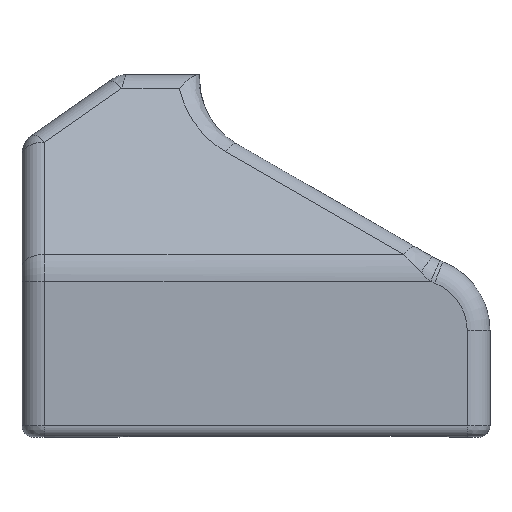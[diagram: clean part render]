
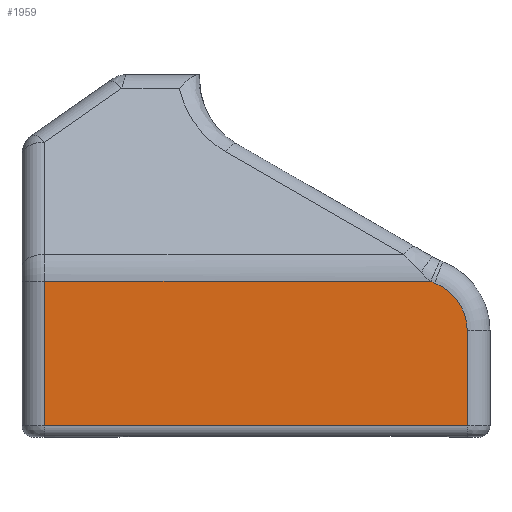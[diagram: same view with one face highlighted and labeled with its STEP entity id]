
A CAD part, left-side view. The second image highlights one B-rep face of the part: STEP entity #1959.
In plain terms, the highlighted planar face has unit normal (-1, 0, 0).
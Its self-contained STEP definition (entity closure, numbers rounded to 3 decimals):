
#72=PLANE('',#2136);
#104=LINE('',#2942,#241);
#123=LINE('',#3056,#260);
#142=LINE('',#3189,#279);
#143=LINE('',#3194,#280);
#241=VECTOR('',#2320,10.);
#260=VECTOR('',#2385,10.);
#279=VECTOR('',#2480,10.);
#280=VECTOR('',#2485,10.);
#490=FACE_OUTER_BOUND('',#613,.T.);
#613=EDGE_LOOP('',(#1442,#1443,#1444,#1445,#1446,#1447));
#750=CIRCLE('',#2137,4.5);
#751=CIRCLE('',#2138,8.5);
#826=VERTEX_POINT('',#2926);
#830=VERTEX_POINT('',#2940);
#857=VERTEX_POINT('',#3055);
#883=VERTEX_POINT('',#3188);
#884=VERTEX_POINT('',#3190);
#885=VERTEX_POINT('',#3192);
#1013=EDGE_CURVE('',#830,#826,#104,.T.);
#1051=EDGE_CURVE('',#826,#857,#123,.T.);
#1094=EDGE_CURVE('',#883,#830,#142,.T.);
#1095=EDGE_CURVE('',#884,#883,#750,.T.);
#1096=EDGE_CURVE('',#885,#884,#751,.T.);
#1097=EDGE_CURVE('',#857,#885,#143,.T.);
#1442=ORIENTED_EDGE('',*,*,#1013,.F.);
#1443=ORIENTED_EDGE('',*,*,#1094,.F.);
#1444=ORIENTED_EDGE('',*,*,#1095,.F.);
#1445=ORIENTED_EDGE('',*,*,#1096,.F.);
#1446=ORIENTED_EDGE('',*,*,#1097,.F.);
#1447=ORIENTED_EDGE('',*,*,#1051,.F.);
#1959=ADVANCED_FACE('',(#490),#72,.T.);
#2136=AXIS2_PLACEMENT_3D('',#3187,#2478,#2479);
#2137=AXIS2_PLACEMENT_3D('',#3191,#2481,#2482);
#2138=AXIS2_PLACEMENT_3D('',#3193,#2483,#2484);
#2320=DIRECTION('',(0.,1.,0.));
#2385=DIRECTION('',(0.,0.,1.));
#2478=DIRECTION('center_axis',(-1.,0.,0.));
#2479=DIRECTION('ref_axis',(0.,-1.,0.));
#2480=DIRECTION('',(0.,0.,-1.));
#2481=DIRECTION('center_axis',(1.,0.,0.));
#2482=DIRECTION('ref_axis',(0.,-0.934,0.358));
#2483=DIRECTION('center_axis',(-1.,0.,0.));
#2484=DIRECTION('ref_axis',(0.,0.361,-0.933));
#2485=DIRECTION('',(0.,-1.,0.));
#2926=CARTESIAN_POINT('',(-3.,36.2,1.));
#2940=CARTESIAN_POINT('',(-3.,-1.,1.));
#2942=CARTESIAN_POINT('',(-3.,23.4,1.));
#3055=CARTESIAN_POINT('',(-3.,36.2,13.718));
#3056=CARTESIAN_POINT('',(-3.,36.2,0.));
#3187=CARTESIAN_POINT('Origin',(-3.,32.2,0.));
#3188=CARTESIAN_POINT('',(-3.,-1.,9.376));
#3189=CARTESIAN_POINT('',(-3.,-1.,0.));
#3190=CARTESIAN_POINT('',(-3.,1.876,13.573));
#3191=CARTESIAN_POINT('Origin',(-3.,3.5,9.376));
#3192=CARTESIAN_POINT('',(-3.,2.227,13.718));
#3193=CARTESIAN_POINT('Origin',(-3.,-1.192,21.5));
#3194=CARTESIAN_POINT('',(-3.,32.2,13.718));
